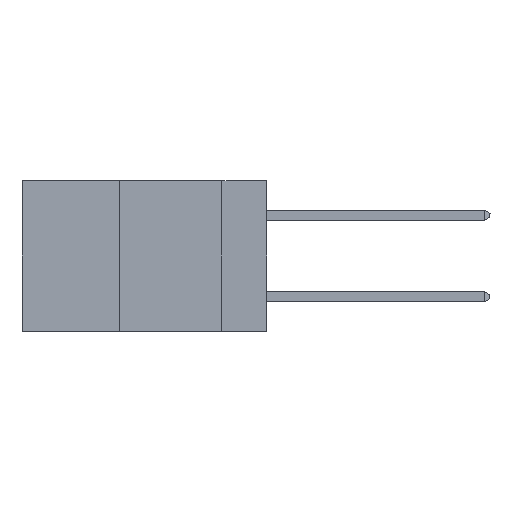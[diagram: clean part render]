
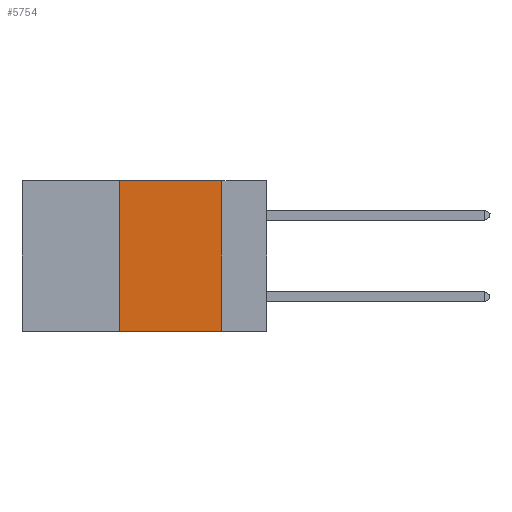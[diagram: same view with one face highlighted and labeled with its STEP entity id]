
A CAD part, left-side view. The second image highlights one B-rep face of the part: STEP entity #5754.
In plain terms, the highlighted planar face has unit normal (-1, 0, 0).
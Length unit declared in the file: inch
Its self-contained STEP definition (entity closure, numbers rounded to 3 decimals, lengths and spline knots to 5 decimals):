
#703 = DIRECTION ( 'NONE',  ( 1., 0., 0. ) ) ;
#877 = LINE ( 'NONE', #3041, #23279 ) ;
#2313 = DIRECTION ( 'NONE',  ( 0., 0., 1. ) ) ;
#2615 = ORIENTED_EDGE ( 'NONE', *, *, #9992, .F. ) ;
#3041 = CARTESIAN_POINT ( 'NONE',  ( 0., 0.6, 0. ) ) ;
#3288 = DIRECTION ( 'NONE',  ( 0., -1., 0. ) ) ;
#4278 = CARTESIAN_POINT ( 'NONE',  ( 0., 0.6, 0. ) ) ;
#5333 = DIRECTION ( 'NONE',  ( 0., -1., 0. ) ) ;
#5754 = ADVANCED_FACE ( 'NONE', ( #21898 ), #18106, .F. ) ;
#5990 = LINE ( 'NONE', #14158, #12181 ) ;
#7155 = CARTESIAN_POINT ( 'NONE',  ( 0., 0.36, 0. ) ) ;
#8095 = ORIENTED_EDGE ( 'NONE', *, *, #22577, .F. ) ;
#8413 = VERTEX_POINT ( 'NONE', #7155 ) ;
#9554 = LINE ( 'NONE', #21077, #21080 ) ;
#9871 = DIRECTION ( 'NONE',  ( 0., 0., -1. ) ) ;
#9952 = ORIENTED_EDGE ( 'NONE', *, *, #15565, .T. ) ;
#9992 = EDGE_CURVE ( 'NONE', #22566, #8413, #5990, .T. ) ;
#11090 = LINE ( 'NONE', #15027, #18776 ) ;
#11573 = AXIS2_PLACEMENT_3D ( 'NONE', #4278, #703, #9871 ) ;
#12181 = VECTOR ( 'NONE', #2313, 39.37008 ) ;
#14158 = CARTESIAN_POINT ( 'NONE',  ( 0., 0.36, 0. ) ) ;
#15027 = CARTESIAN_POINT ( 'NONE',  ( 0., 0.6, -0.37 ) ) ;
#15565 = EDGE_CURVE ( 'NONE', #22566, #22376, #11090, .T. ) ;
#16805 = EDGE_CURVE ( 'NONE', #8413, #24579, #877, .T. ) ;
#17761 = CARTESIAN_POINT ( 'NONE',  ( 0., 0.11, 0. ) ) ;
#18106 = PLANE ( 'NONE',  #11573 ) ;
#18713 = EDGE_LOOP ( 'NONE', ( #8095, #21157, #2615, #9952 ) ) ;
#18776 = VECTOR ( 'NONE', #5333, 39.37008 ) ;
#20745 = CARTESIAN_POINT ( 'NONE',  ( 0., 0.11, -0.37 ) ) ;
#21077 = CARTESIAN_POINT ( 'NONE',  ( 0., 0.11, 0. ) ) ;
#21080 = VECTOR ( 'NONE', #23251, 39.37008 ) ;
#21157 = ORIENTED_EDGE ( 'NONE', *, *, #16805, .F. ) ;
#21898 = FACE_OUTER_BOUND ( 'NONE', #18713, .T. ) ;
#22376 = VERTEX_POINT ( 'NONE', #20745 ) ;
#22566 = VERTEX_POINT ( 'NONE', #24537 ) ;
#22577 = EDGE_CURVE ( 'NONE', #24579, #22376, #9554, .T. ) ;
#23251 = DIRECTION ( 'NONE',  ( 0., 0., -1. ) ) ;
#23279 = VECTOR ( 'NONE', #3288, 39.37008 ) ;
#24537 = CARTESIAN_POINT ( 'NONE',  ( 0., 0.36, -0.37 ) ) ;
#24579 = VERTEX_POINT ( 'NONE', #17761 ) ;
